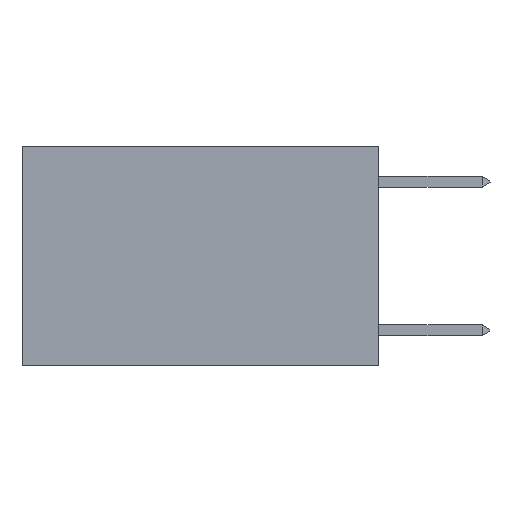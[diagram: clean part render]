
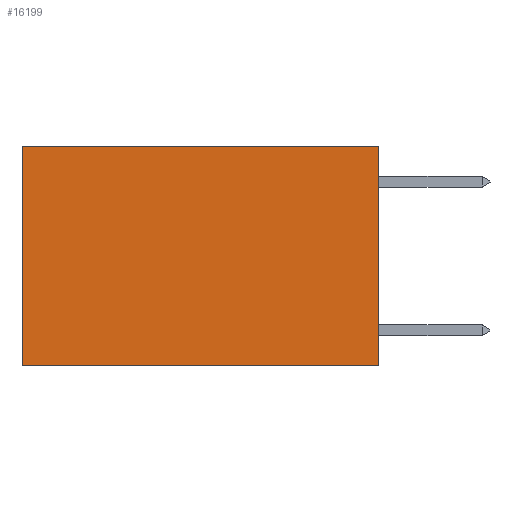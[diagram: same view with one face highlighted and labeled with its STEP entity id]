
A CAD part, left-side view. The second image highlights one B-rep face of the part: STEP entity #16199.
In plain terms, the highlighted planar face has unit normal (-1, 0, 0).
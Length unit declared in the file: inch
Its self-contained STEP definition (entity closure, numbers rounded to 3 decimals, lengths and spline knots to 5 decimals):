
#41 = ORIENTED_EDGE ( 'NONE', *, *, #5374, .F. ) ;
#162 = DIRECTION ( 'NONE',  ( 0., 0., -1. ) ) ;
#400 = EDGE_CURVE ( 'NONE', #14740, #9447, #5818, .T. ) ;
#1569 = ORIENTED_EDGE ( 'NONE', *, *, #11752, .F. ) ;
#1754 = CARTESIAN_POINT ( 'NONE',  ( 0.2625, 0.6, 0. ) ) ;
#1853 = LINE ( 'NONE', #5672, #7794 ) ;
#2351 = CARTESIAN_POINT ( 'NONE',  ( 0.2625, 0., 0. ) ) ;
#2839 = VECTOR ( 'NONE', #11217, 39.37008 ) ;
#3113 = EDGE_LOOP ( 'NONE', ( #11705, #41, #1569, #9050 ) ) ;
#3176 = DIRECTION ( 'NONE',  ( 0., 0., -1. ) ) ;
#4314 = CARTESIAN_POINT ( 'NONE',  ( 0.2625, 0.6, -0.37 ) ) ;
#4342 = EDGE_CURVE ( 'NONE', #14772, #14740, #10377, .T. ) ;
#4370 = CARTESIAN_POINT ( 'NONE',  ( 0.2625, 0.6, 0. ) ) ;
#5374 = EDGE_CURVE ( 'NONE', #7606, #9447, #11736, .T. ) ;
#5672 = CARTESIAN_POINT ( 'NONE',  ( 0.2625, 0., 0. ) ) ;
#5818 = LINE ( 'NONE', #4370, #2839 ) ;
#5867 = FACE_OUTER_BOUND ( 'NONE', #3113, .T. ) ;
#6183 = DIRECTION ( 'NONE',  ( 0., 1., 0. ) ) ;
#6269 = AXIS2_PLACEMENT_3D ( 'NONE', #10206, #7738, #162 ) ;
#6459 = PLANE ( 'NONE',  #6269 ) ;
#7606 = VERTEX_POINT ( 'NONE', #10716 ) ;
#7738 = DIRECTION ( 'NONE',  ( 1., 0., 0. ) ) ;
#7794 = VECTOR ( 'NONE', #3176, 39.37008 ) ;
#8119 = CARTESIAN_POINT ( 'NONE',  ( 0.2625, 0., 0. ) ) ;
#9050 = ORIENTED_EDGE ( 'NONE', *, *, #4342, .T. ) ;
#9447 = VERTEX_POINT ( 'NONE', #4314 ) ;
#9982 = VECTOR ( 'NONE', #6183, 39.37008 ) ;
#10206 = CARTESIAN_POINT ( 'NONE',  ( 0.2625, 0., 0. ) ) ;
#10377 = LINE ( 'NONE', #2351, #9982 ) ;
#10716 = CARTESIAN_POINT ( 'NONE',  ( 0.2625, 0., -0.37 ) ) ;
#11217 = DIRECTION ( 'NONE',  ( 0., 0., -1. ) ) ;
#11705 = ORIENTED_EDGE ( 'NONE', *, *, #400, .T. ) ;
#11736 = LINE ( 'NONE', #11793, #15513 ) ;
#11752 = EDGE_CURVE ( 'NONE', #14772, #7606, #1853, .T. ) ;
#11793 = CARTESIAN_POINT ( 'NONE',  ( 0.2625, 0., -0.37 ) ) ;
#13009 = DIRECTION ( 'NONE',  ( 0., 1., 0. ) ) ;
#14740 = VERTEX_POINT ( 'NONE', #1754 ) ;
#14772 = VERTEX_POINT ( 'NONE', #8119 ) ;
#15513 = VECTOR ( 'NONE', #13009, 39.37008 ) ;
#16199 = ADVANCED_FACE ( 'NONE', ( #5867 ), #6459, .F. ) ;
